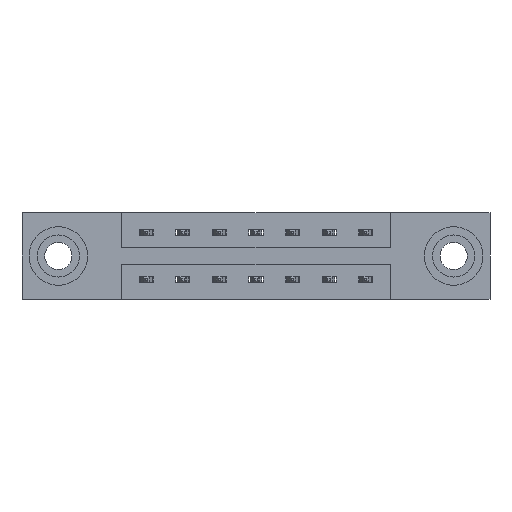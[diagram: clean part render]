
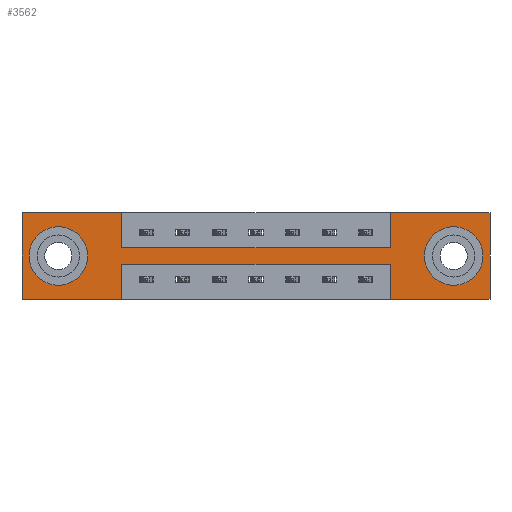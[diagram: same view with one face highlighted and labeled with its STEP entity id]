
A CAD part, front view. The second image highlights one B-rep face of the part: STEP entity #3562.
In plain terms, the highlighted planar face has unit normal (0, -1, 0).
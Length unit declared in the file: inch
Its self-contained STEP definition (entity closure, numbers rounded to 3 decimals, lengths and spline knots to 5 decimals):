
#51 = DIRECTION ( 'NONE',  ( 0., 0., 1. ) ) ;
#127 = VERTEX_POINT ( 'NONE', #8946 ) ;
#191 = ORIENTED_EDGE ( 'NONE', *, *, #4170, .F. ) ;
#219 = CARTESIAN_POINT ( 'NONE',  ( 1.573, 0., 0. ) ) ;
#313 = CIRCLE ( 'NONE', #3276, 0.078 ) ;
#406 = FACE_OUTER_BOUND ( 'NONE', #10130, .T. ) ;
#431 = EDGE_CURVE ( 'NONE', #4798, #9057, #9257, .T. ) ;
#505 = CARTESIAN_POINT ( 'NONE',  ( 0., 0., -0.37 ) ) ;
#651 = EDGE_CURVE ( 'NONE', #9057, #5676, #3066, .T. ) ;
#874 = VERTEX_POINT ( 'NONE', #10022 ) ;
#948 = CARTESIAN_POINT ( 'NONE',  ( 0.155, 0., -0.185 ) ) ;
#1053 = DIRECTION ( 'NONE',  ( 0., 0., 1. ) ) ;
#1196 = ORIENTED_EDGE ( 'NONE', *, *, #9220, .T. ) ;
#1276 = CARTESIAN_POINT ( 'NONE',  ( 0.425, 0., -0.22 ) ) ;
#1306 = VERTEX_POINT ( 'NONE', #5161 ) ;
#1421 = VECTOR ( 'NONE', #9767, 39.37008 ) ;
#1450 = FACE_BOUND ( 'NONE', #1706, .T. ) ;
#1667 = DIRECTION ( 'NONE',  ( 0., 1., 0. ) ) ;
#1706 = EDGE_LOOP ( 'NONE', ( #1196, #8539 ) ) ;
#1746 = DIRECTION ( 'NONE',  ( 0., 0., 1. ) ) ;
#1801 = DIRECTION ( 'NONE',  ( -1., 0., 0. ) ) ;
#1841 = VECTOR ( 'NONE', #1801, 39.37008 ) ;
#1960 = EDGE_CURVE ( 'NONE', #2907, #3136, #6503, .T. ) ;
#2008 = ORIENTED_EDGE ( 'NONE', *, *, #3458, .F. ) ;
#2039 = EDGE_LOOP ( 'NONE', ( #5390, #7973 ) ) ;
#2115 = EDGE_CURVE ( 'NONE', #5676, #4431, #2130, .T. ) ;
#2130 = LINE ( 'NONE', #1276, #4575 ) ;
#2207 = EDGE_CURVE ( 'NONE', #9993, #874, #313, .T. ) ;
#2251 = DIRECTION ( 'NONE',  ( -1., 0., 0. ) ) ;
#2352 = VECTOR ( 'NONE', #8102, 39.37008 ) ;
#2359 = VECTOR ( 'NONE', #10534, 39.37008 ) ;
#2392 = VECTOR ( 'NONE', #1053, 39.37008 ) ;
#2455 = ORIENTED_EDGE ( 'NONE', *, *, #651, .F. ) ;
#2545 = CARTESIAN_POINT ( 'NONE',  ( 0.425, 0., -0.22 ) ) ;
#2647 = DIRECTION ( 'NONE',  ( 0., -1., 0. ) ) ;
#2704 = CARTESIAN_POINT ( 'NONE',  ( 1.998, 0., 0. ) ) ;
#2855 = LINE ( 'NONE', #4150, #1841 ) ;
#2907 = VERTEX_POINT ( 'NONE', #5648 ) ;
#3017 = CARTESIAN_POINT ( 'NONE',  ( 0.425, 0., 0. ) ) ;
#3060 = LINE ( 'NONE', #7006, #5884 ) ;
#3066 = LINE ( 'NONE', #5783, #8092 ) ;
#3136 = VERTEX_POINT ( 'NONE', #2704 ) ;
#3276 = AXIS2_PLACEMENT_3D ( 'NONE', #3418, #8370, #5992 ) ;
#3382 = FACE_BOUND ( 'NONE', #2039, .T. ) ;
#3418 = CARTESIAN_POINT ( 'NONE',  ( 0.155, 0., -0.185 ) ) ;
#3458 = EDGE_CURVE ( 'NONE', #5035, #127, #5568, .T. ) ;
#3553 = VERTEX_POINT ( 'NONE', #8427 ) ;
#3562 = ADVANCED_FACE ( 'NONE', ( #3382, #1450, #406 ), #7501, .T. ) ;
#3736 = AXIS2_PLACEMENT_3D ( 'NONE', #948, #9075, #1746 ) ;
#3769 = ORIENTED_EDGE ( 'NONE', *, *, #4426, .F. ) ;
#3873 = EDGE_CURVE ( 'NONE', #6077, #4261, #9923, .T. ) ;
#4063 = CARTESIAN_POINT ( 'NONE',  ( 0.155, 0., -0.263 ) ) ;
#4094 = CARTESIAN_POINT ( 'NONE',  ( 0.425, 0., -0.15 ) ) ;
#4150 = CARTESIAN_POINT ( 'NONE',  ( 0., 0., -0.37 ) ) ;
#4170 = EDGE_CURVE ( 'NONE', #127, #5311, #8266, .T. ) ;
#4244 = ORIENTED_EDGE ( 'NONE', *, *, #4821, .F. ) ;
#4261 = VERTEX_POINT ( 'NONE', #10573 ) ;
#4268 = LINE ( 'NONE', #4939, #2352 ) ;
#4373 = CARTESIAN_POINT ( 'NONE',  ( 0., 0., 0. ) ) ;
#4392 = AXIS2_PLACEMENT_3D ( 'NONE', #5089, #2647, #8392 ) ;
#4426 = EDGE_CURVE ( 'NONE', #1306, #5035, #2855, .T. ) ;
#4431 = VERTEX_POINT ( 'NONE', #2545 ) ;
#4575 = VECTOR ( 'NONE', #9513, 39.37008 ) ;
#4619 = VECTOR ( 'NONE', #2251, 39.37008 ) ;
#4667 = CARTESIAN_POINT ( 'NONE',  ( 0.425, 0., -0.15 ) ) ;
#4798 = VERTEX_POINT ( 'NONE', #6449 ) ;
#4821 = EDGE_CURVE ( 'NONE', #4431, #1306, #9916, .T. ) ;
#4822 = AXIS2_PLACEMENT_3D ( 'NONE', #6584, #1667, #7636 ) ;
#4847 = CARTESIAN_POINT ( 'NONE',  ( 1.843, 0., -0.185 ) ) ;
#4939 = CARTESIAN_POINT ( 'NONE',  ( 1.998, 0., 0. ) ) ;
#4976 = VECTOR ( 'NONE', #5200, 39.37008 ) ;
#5035 = VERTEX_POINT ( 'NONE', #5865 ) ;
#5089 = CARTESIAN_POINT ( 'NONE',  ( 0., 0., -0.37 ) ) ;
#5111 = ORIENTED_EDGE ( 'NONE', *, *, #7733, .F. ) ;
#5161 = CARTESIAN_POINT ( 'NONE',  ( 0.425, 0., -0.37 ) ) ;
#5200 = DIRECTION ( 'NONE',  ( 1., 0., 0. ) ) ;
#5311 = VERTEX_POINT ( 'NONE', #3017 ) ;
#5390 = ORIENTED_EDGE ( 'NONE', *, *, #7073, .T. ) ;
#5568 = LINE ( 'NONE', #8226, #9434 ) ;
#5633 = CARTESIAN_POINT ( 'NONE',  ( 0., 0., 0. ) ) ;
#5648 = CARTESIAN_POINT ( 'NONE',  ( 1.573, 0., 0. ) ) ;
#5676 = VERTEX_POINT ( 'NONE', #6875 ) ;
#5771 = ORIENTED_EDGE ( 'NONE', *, *, #431, .F. ) ;
#5783 = CARTESIAN_POINT ( 'NONE',  ( 1.573, 0., -0.37 ) ) ;
#5865 = CARTESIAN_POINT ( 'NONE',  ( 0., 0., -0.37 ) ) ;
#5884 = VECTOR ( 'NONE', #10180, 39.37008 ) ;
#5992 = DIRECTION ( 'NONE',  ( 0., 0., 1. ) ) ;
#6041 = EDGE_CURVE ( 'NONE', #5311, #10535, #3060, .T. ) ;
#6077 = VERTEX_POINT ( 'NONE', #8551 ) ;
#6449 = CARTESIAN_POINT ( 'NONE',  ( 1.998, 0., -0.37 ) ) ;
#6503 = LINE ( 'NONE', #4373, #4976 ) ;
#6584 = CARTESIAN_POINT ( 'NONE',  ( 1.843, 0., -0.185 ) ) ;
#6593 = DIRECTION ( 'NONE',  ( 0., 0., 1. ) ) ;
#6875 = CARTESIAN_POINT ( 'NONE',  ( 1.573, 0., -0.22 ) ) ;
#7006 = CARTESIAN_POINT ( 'NONE',  ( 0.425, 0., 0. ) ) ;
#7073 = EDGE_CURVE ( 'NONE', #4261, #6077, #7795, .T. ) ;
#7103 = ORIENTED_EDGE ( 'NONE', *, *, #7273, .F. ) ;
#7154 = LINE ( 'NONE', #219, #2392 ) ;
#7270 = DIRECTION ( 'NONE',  ( 1., 0., 0. ) ) ;
#7273 = EDGE_CURVE ( 'NONE', #3553, #2907, #7154, .T. ) ;
#7322 = DIRECTION ( 'NONE',  ( 0., 1., 0. ) ) ;
#7501 = PLANE ( 'NONE',  #4392 ) ;
#7636 = DIRECTION ( 'NONE',  ( 0., 0., -1. ) ) ;
#7733 = EDGE_CURVE ( 'NONE', #10535, #3553, #8940, .T. ) ;
#7795 = CIRCLE ( 'NONE', #9728, 0.078 ) ;
#7973 = ORIENTED_EDGE ( 'NONE', *, *, #3873, .T. ) ;
#8092 = VECTOR ( 'NONE', #6593, 39.37008 ) ;
#8102 = DIRECTION ( 'NONE',  ( 0., 0., -1. ) ) ;
#8173 = VECTOR ( 'NONE', #7270, 39.37008 ) ;
#8226 = CARTESIAN_POINT ( 'NONE',  ( 0., 0., 0. ) ) ;
#8266 = LINE ( 'NONE', #5633, #2359 ) ;
#8370 = DIRECTION ( 'NONE',  ( 0., 1., 0. ) ) ;
#8383 = CIRCLE ( 'NONE', #3736, 0.078 ) ;
#8392 = DIRECTION ( 'NONE',  ( 0., 0., -1. ) ) ;
#8426 = ORIENTED_EDGE ( 'NONE', *, *, #2115, .F. ) ;
#8427 = CARTESIAN_POINT ( 'NONE',  ( 1.573, 0., -0.15 ) ) ;
#8539 = ORIENTED_EDGE ( 'NONE', *, *, #2207, .T. ) ;
#8551 = CARTESIAN_POINT ( 'NONE',  ( 1.843, 0., -0.263 ) ) ;
#8828 = CARTESIAN_POINT ( 'NONE',  ( 0.425, 0., -0.37 ) ) ;
#8914 = ORIENTED_EDGE ( 'NONE', *, *, #6041, .F. ) ;
#8940 = LINE ( 'NONE', #4094, #8173 ) ;
#8946 = CARTESIAN_POINT ( 'NONE',  ( 0., 0., 0. ) ) ;
#9057 = VERTEX_POINT ( 'NONE', #9795 ) ;
#9075 = DIRECTION ( 'NONE',  ( 0., 1., 0. ) ) ;
#9134 = ORIENTED_EDGE ( 'NONE', *, *, #9875, .F. ) ;
#9220 = EDGE_CURVE ( 'NONE', #874, #9993, #8383, .T. ) ;
#9257 = LINE ( 'NONE', #505, #4619 ) ;
#9434 = VECTOR ( 'NONE', #51, 39.37008 ) ;
#9513 = DIRECTION ( 'NONE',  ( -1., 0., 0. ) ) ;
#9728 = AXIS2_PLACEMENT_3D ( 'NONE', #4847, #7322, #10558 ) ;
#9767 = DIRECTION ( 'NONE',  ( 0., 0., -1. ) ) ;
#9795 = CARTESIAN_POINT ( 'NONE',  ( 1.573, 0., -0.37 ) ) ;
#9875 = EDGE_CURVE ( 'NONE', #3136, #4798, #4268, .T. ) ;
#9916 = LINE ( 'NONE', #8828, #1421 ) ;
#9923 = CIRCLE ( 'NONE', #4822, 0.078 ) ;
#9955 = ORIENTED_EDGE ( 'NONE', *, *, #1960, .F. ) ;
#9993 = VERTEX_POINT ( 'NONE', #4063 ) ;
#10022 = CARTESIAN_POINT ( 'NONE',  ( 0.155, 0., -0.107 ) ) ;
#10130 = EDGE_LOOP ( 'NONE', ( #4244, #8426, #2455, #5771, #9134, #9955, #7103, #5111, #8914, #191, #2008, #3769 ) ) ;
#10180 = DIRECTION ( 'NONE',  ( 0., 0., -1. ) ) ;
#10534 = DIRECTION ( 'NONE',  ( 1., 0., 0. ) ) ;
#10535 = VERTEX_POINT ( 'NONE', #4667 ) ;
#10558 = DIRECTION ( 'NONE',  ( 0., 0., -1. ) ) ;
#10573 = CARTESIAN_POINT ( 'NONE',  ( 1.843, 0., -0.107 ) ) ;
